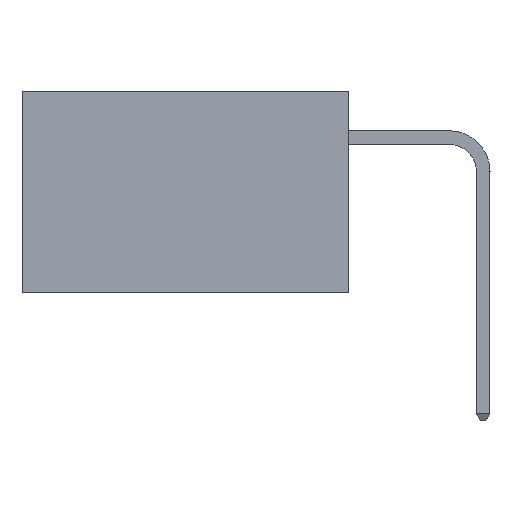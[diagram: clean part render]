
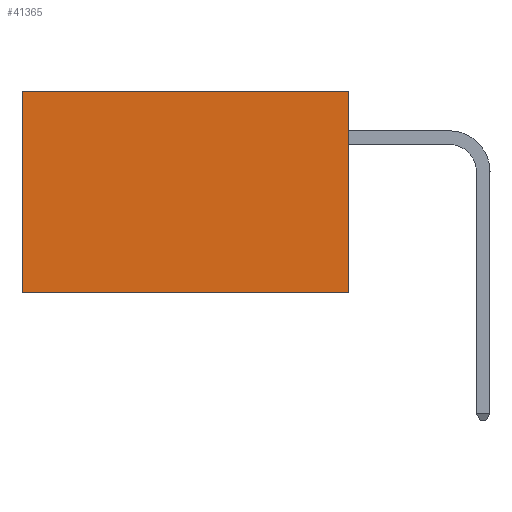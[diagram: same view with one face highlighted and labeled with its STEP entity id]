
A CAD part, left-side view. The second image highlights one B-rep face of the part: STEP entity #41365.
In plain terms, the highlighted planar face has unit normal (-1, 0, 0).
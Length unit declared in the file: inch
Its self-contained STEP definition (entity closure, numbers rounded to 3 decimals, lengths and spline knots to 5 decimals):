
#289 = VERTEX_POINT ( 'NONE', #41113 ) ;
#1838 = ORIENTED_EDGE ( 'NONE', *, *, #2973, .F. ) ;
#2016 = VECTOR ( 'NONE', #43174, 39.37008 ) ;
#2973 = EDGE_CURVE ( 'NONE', #289, #36603, #30901, .T. ) ;
#3465 = CARTESIAN_POINT ( 'NONE',  ( 0.2875, 0., 0. ) ) ;
#3523 = CARTESIAN_POINT ( 'NONE',  ( 0.2875, 0.6, 0. ) ) ;
#4523 = LINE ( 'NONE', #3523, #5105 ) ;
#5105 = VECTOR ( 'NONE', #41778, 39.37008 ) ;
#6083 = ORIENTED_EDGE ( 'NONE', *, *, #42968, .T. ) ;
#9259 = CARTESIAN_POINT ( 'NONE',  ( 0.2875, 0.6, 0. ) ) ;
#10790 = DIRECTION ( 'NONE',  ( 0., 1., 0. ) ) ;
#12013 = DIRECTION ( 'NONE',  ( 0., 0., -1. ) ) ;
#13774 = FACE_OUTER_BOUND ( 'NONE', #32980, .T. ) ;
#14732 = VECTOR ( 'NONE', #10790, 39.37008 ) ;
#15640 = CARTESIAN_POINT ( 'NONE',  ( 0.2875, 0., -0.37 ) ) ;
#16832 = DIRECTION ( 'NONE',  ( 0., 0., -1. ) ) ;
#17667 = VECTOR ( 'NONE', #16832, 39.37008 ) ;
#20018 = VERTEX_POINT ( 'NONE', #9259 ) ;
#20487 = VERTEX_POINT ( 'NONE', #44887 ) ;
#20693 = LINE ( 'NONE', #3465, #14732 ) ;
#21450 = LINE ( 'NONE', #41294, #17667 ) ;
#25974 = EDGE_CURVE ( 'NONE', #20018, #36603, #4523, .T. ) ;
#26272 = CARTESIAN_POINT ( 'NONE',  ( 0.2875, 0.6, -0.37 ) ) ;
#26311 = EDGE_CURVE ( 'NONE', #20487, #289, #21450, .T. ) ;
#26810 = AXIS2_PLACEMENT_3D ( 'NONE', #39570, #32338, #12013 ) ;
#30901 = LINE ( 'NONE', #15640, #2016 ) ;
#32338 = DIRECTION ( 'NONE',  ( 1., 0., 0. ) ) ;
#32980 = EDGE_LOOP ( 'NONE', ( #36684, #1838, #44309, #6083 ) ) ;
#36603 = VERTEX_POINT ( 'NONE', #26272 ) ;
#36684 = ORIENTED_EDGE ( 'NONE', *, *, #25974, .T. ) ;
#39570 = CARTESIAN_POINT ( 'NONE',  ( 0.2875, 0., 0. ) ) ;
#41113 = CARTESIAN_POINT ( 'NONE',  ( 0.2875, 0., -0.37 ) ) ;
#41294 = CARTESIAN_POINT ( 'NONE',  ( 0.2875, 0., 0. ) ) ;
#41365 = ADVANCED_FACE ( 'NONE', ( #13774 ), #42912, .F. ) ;
#41778 = DIRECTION ( 'NONE',  ( 0., 0., -1. ) ) ;
#42912 = PLANE ( 'NONE',  #26810 ) ;
#42968 = EDGE_CURVE ( 'NONE', #20487, #20018, #20693, .T. ) ;
#43174 = DIRECTION ( 'NONE',  ( 0., 1., 0. ) ) ;
#44309 = ORIENTED_EDGE ( 'NONE', *, *, #26311, .F. ) ;
#44887 = CARTESIAN_POINT ( 'NONE',  ( 0.2875, 0., 0. ) ) ;
